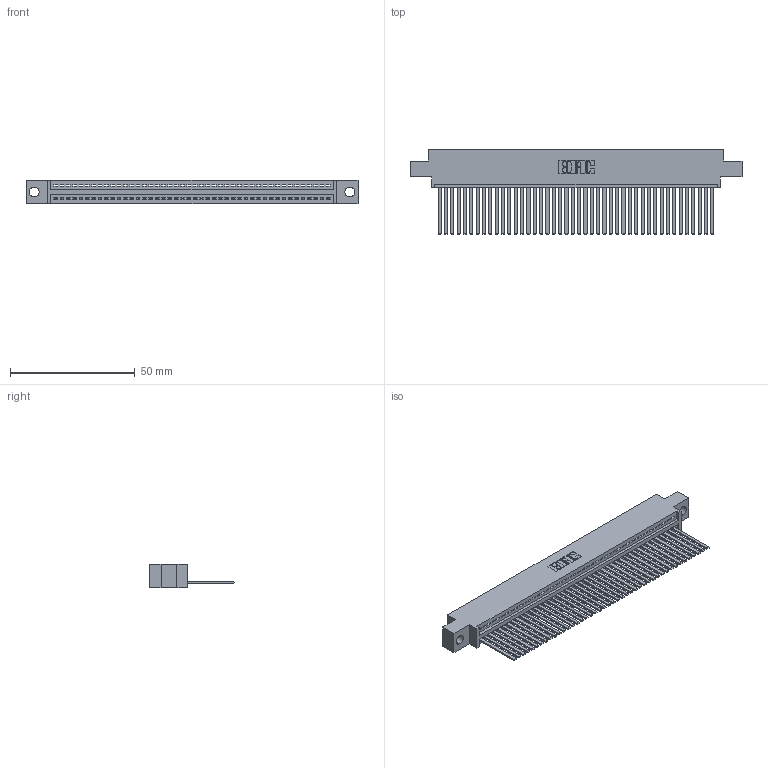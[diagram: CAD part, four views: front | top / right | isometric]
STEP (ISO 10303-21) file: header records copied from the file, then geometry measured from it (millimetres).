
FILE_DESCRIPTION (( 'STEP AP203' ), '1' );
FILE_NAME ('395-044-544-604.STEP', '2018-11-15T21:40:06', ( '' ), ( '' ), 'SwSTEP 2.0', 'SolidWorks 2016', '' );
FILE_SCHEMA (( 'CONFIG_CONTROL_DESIGN' ));
Length unit declared in the file: inch
Products named in the file (3): 395-044-544-604; 345-292-001_345-293-144; 345 Part_0.170 Offset - 0.156 Dia-TH
Assembly tree (45 placements, depth 2):
  395-044-544-604
    345 Part_0.170 Offset - 0.156 Dia-TH
    345-292-001_345-293-144  x44
Bounding box: 132.97 x 33.96 x 9.4 mm (x, y, z)
Volume: 12954.2 mm3; surface area: 18707.3 mm2
Topology: 45 solids, 45 shells, 2418 faces, 7305 edges, 4810 vertices
Faces by surface type: plane 1668, cylinder 750
Entity records: 32797 total; most frequent: CARTESIAN_POINT 5688, ORIENTED_EDGE 5666, DIRECTION 4961, EDGE_CURVE 2833, LINE 2529, VECTOR 2529, VERTEX_POINT 1886, AXIS2_PLACEMENT_3D 1216
